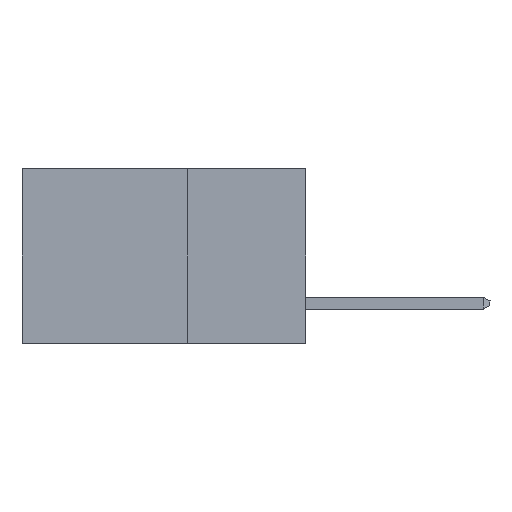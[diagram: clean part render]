
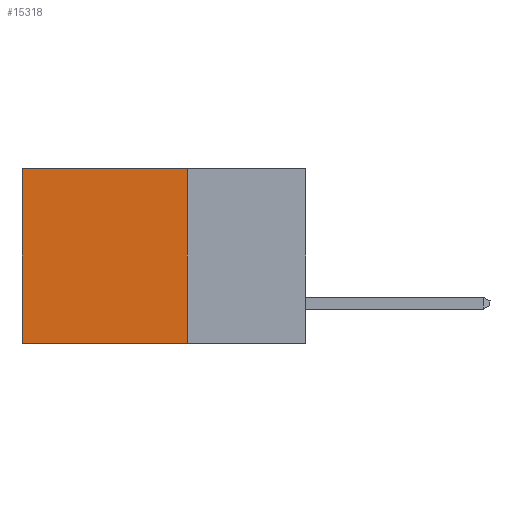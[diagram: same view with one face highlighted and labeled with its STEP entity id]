
A CAD part, left-side view. The second image highlights one B-rep face of the part: STEP entity #15318.
In plain terms, the highlighted planar face has unit normal (-1, 0, 0).
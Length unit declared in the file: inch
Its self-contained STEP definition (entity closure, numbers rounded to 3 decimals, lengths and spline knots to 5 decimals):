
#409 = EDGE_LOOP ( 'NONE', ( #16098, #6966, #27482, #3214 ) ) ;
#1460 = EDGE_CURVE ( 'NONE', #10116, #7788, #5014, .T. ) ;
#1796 = DIRECTION ( 'NONE',  ( 0., 0., -1. ) ) ;
#2245 = CARTESIAN_POINT ( 'NONE',  ( 0.298, 0.6, -0.37 ) ) ;
#2861 = VECTOR ( 'NONE', #27271, 39.37008 ) ;
#3214 = ORIENTED_EDGE ( 'NONE', *, *, #25743, .T. ) ;
#5014 = LINE ( 'NONE', #27371, #2861 ) ;
#6966 = ORIENTED_EDGE ( 'NONE', *, *, #7829, .F. ) ;
#7788 = VERTEX_POINT ( 'NONE', #2245 ) ;
#7829 = EDGE_CURVE ( 'NONE', #21698, #7788, #24273, .T. ) ;
#8511 = DIRECTION ( 'NONE',  ( 1., 0., 0. ) ) ;
#10116 = VERTEX_POINT ( 'NONE', #13606 ) ;
#11247 = DIRECTION ( 'NONE',  ( 0., 1., 0. ) ) ;
#11351 = CARTESIAN_POINT ( 'NONE',  ( 0.298, 0.25, 0. ) ) ;
#11715 = CARTESIAN_POINT ( 'NONE',  ( 0.298, 0.25, -0.37 ) ) ;
#12162 = VECTOR ( 'NONE', #1796, 39.37008 ) ;
#12806 = CARTESIAN_POINT ( 'NONE',  ( 0.298, 0.25, 0. ) ) ;
#13606 = CARTESIAN_POINT ( 'NONE',  ( 0.298, 0.6, 0. ) ) ;
#15245 = CARTESIAN_POINT ( 'NONE',  ( 0.298, 0.25, 0. ) ) ;
#15318 = ADVANCED_FACE ( 'NONE', ( #21853 ), #17658, .F. ) ;
#15395 = DIRECTION ( 'NONE',  ( 0., 1., 0. ) ) ;
#15497 = CARTESIAN_POINT ( 'NONE',  ( 0.298, 0.25, -0.37 ) ) ;
#16098 = ORIENTED_EDGE ( 'NONE', *, *, #1460, .T. ) ;
#16707 = EDGE_CURVE ( 'NONE', #19609, #21698, #27435, .T. ) ;
#17658 = PLANE ( 'NONE',  #22420 ) ;
#17849 = VECTOR ( 'NONE', #15395, 39.37008 ) ;
#18596 = LINE ( 'NONE', #11351, #21093 ) ;
#19609 = VERTEX_POINT ( 'NONE', #12806 ) ;
#19770 = DIRECTION ( 'NONE',  ( 0., 0., -1. ) ) ;
#21093 = VECTOR ( 'NONE', #11247, 39.37008 ) ;
#21698 = VERTEX_POINT ( 'NONE', #11715 ) ;
#21853 = FACE_OUTER_BOUND ( 'NONE', #409, .T. ) ;
#22420 = AXIS2_PLACEMENT_3D ( 'NONE', #26918, #8511, #19770 ) ;
#24273 = LINE ( 'NONE', #15497, #17849 ) ;
#25743 = EDGE_CURVE ( 'NONE', #19609, #10116, #18596, .T. ) ;
#26918 = CARTESIAN_POINT ( 'NONE',  ( 0.298, 0.25, 0. ) ) ;
#27271 = DIRECTION ( 'NONE',  ( 0., 0., -1. ) ) ;
#27371 = CARTESIAN_POINT ( 'NONE',  ( 0.298, 0.6, 0. ) ) ;
#27435 = LINE ( 'NONE', #15245, #12162 ) ;
#27482 = ORIENTED_EDGE ( 'NONE', *, *, #16707, .F. ) ;
